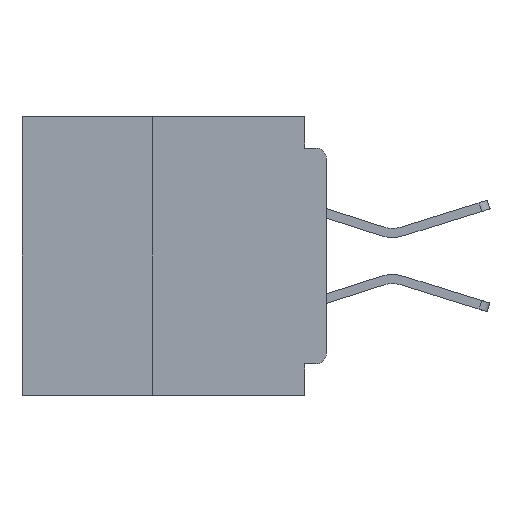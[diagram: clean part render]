
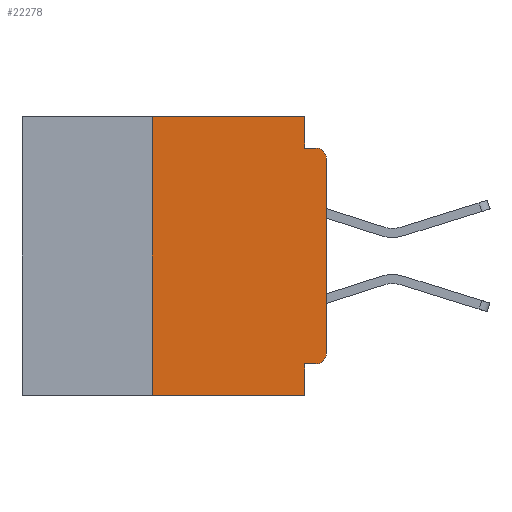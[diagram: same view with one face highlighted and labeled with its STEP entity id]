
A CAD part, left-side view. The second image highlights one B-rep face of the part: STEP entity #22278.
In plain terms, the highlighted planar face has unit normal (-1, 0, 0).
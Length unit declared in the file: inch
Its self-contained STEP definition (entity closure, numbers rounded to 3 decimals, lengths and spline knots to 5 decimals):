
#838 = DIRECTION ( 'NONE',  ( 0., 0., -1. ) ) ;
#1264 = DIRECTION ( 'NONE',  ( -1., 0., 0. ) ) ;
#1279 = VECTOR ( 'NONE', #4984, 39.37008 ) ;
#2149 = VERTEX_POINT ( 'NONE', #19976 ) ;
#2242 = AXIS2_PLACEMENT_3D ( 'NONE', #22116, #1264, #25553 ) ;
#2378 = ORIENTED_EDGE ( 'NONE', *, *, #42520, .T. ) ;
#2770 = VECTOR ( 'NONE', #7471, 39.37008 ) ;
#3563 = CARTESIAN_POINT ( 'NONE',  ( 0., 0., -0.34 ) ) ;
#3921 = CARTESIAN_POINT ( 'NONE',  ( 0., 0., -0.355 ) ) ;
#4330 = ORIENTED_EDGE ( 'NONE', *, *, #10132, .F. ) ;
#4984 = DIRECTION ( 'NONE',  ( 0., -1., 0. ) ) ;
#5129 = DIRECTION ( 'NONE',  ( 1., 0., 0. ) ) ;
#6681 = DIRECTION ( 'NONE',  ( 0., 0., -1. ) ) ;
#6884 = LINE ( 'NONE', #18357, #33269 ) ;
#7471 = DIRECTION ( 'NONE',  ( 0., 1., 0. ) ) ;
#7652 = DIRECTION ( 'NONE',  ( -1., 0., 0. ) ) ;
#9373 = CARTESIAN_POINT ( 'NONE',  ( 0., 0.437, 0. ) ) ;
#9387 = CARTESIAN_POINT ( 'NONE',  ( 0., 0.015, -0.045 ) ) ;
#9843 = ORIENTED_EDGE ( 'NONE', *, *, #18366, .F. ) ;
#10132 = EDGE_CURVE ( 'NONE', #31865, #11910, #21342, .T. ) ;
#10549 = LINE ( 'NONE', #25743, #36832 ) ;
#10996 = EDGE_CURVE ( 'NONE', #33162, #15261, #13133, .T. ) ;
#11572 = LINE ( 'NONE', #27353, #28836 ) ;
#11817 = CARTESIAN_POINT ( 'NONE',  ( 0., 0.437, -0.4 ) ) ;
#11910 = VERTEX_POINT ( 'NONE', #9387 ) ;
#11951 = DIRECTION ( 'NONE',  ( 0., -1., 0. ) ) ;
#12025 = VERTEX_POINT ( 'NONE', #23714 ) ;
#12152 = VECTOR ( 'NONE', #11951, 39.37008 ) ;
#12758 = CARTESIAN_POINT ( 'NONE',  ( 0., 0., 0. ) ) ;
#13133 = LINE ( 'NONE', #3921, #2770 ) ;
#15261 = VERTEX_POINT ( 'NONE', #28541 ) ;
#15314 = ORIENTED_EDGE ( 'NONE', *, *, #25732, .T. ) ;
#15579 = VECTOR ( 'NONE', #16210, 39.37008 ) ;
#15682 = ORIENTED_EDGE ( 'NONE', *, *, #27610, .F. ) ;
#16181 = EDGE_CURVE ( 'NONE', #16954, #34588, #42872, .T. ) ;
#16210 = DIRECTION ( 'NONE',  ( 0., 0., 1. ) ) ;
#16509 = AXIS2_PLACEMENT_3D ( 'NONE', #28320, #7652, #31721 ) ;
#16954 = VERTEX_POINT ( 'NONE', #3563 ) ;
#17645 = ORIENTED_EDGE ( 'NONE', *, *, #38196, .F. ) ;
#18357 = CARTESIAN_POINT ( 'NONE',  ( 0., 0.031, 0. ) ) ;
#18366 = EDGE_CURVE ( 'NONE', #2149, #34542, #10549, .T. ) ;
#18877 = CARTESIAN_POINT ( 'NONE',  ( 0., 0.437, 0. ) ) ;
#19976 = CARTESIAN_POINT ( 'NONE',  ( 0., 0.25, -0.4 ) ) ;
#20251 = CARTESIAN_POINT ( 'NONE',  ( 0., 0.015, -0.355 ) ) ;
#21342 = LINE ( 'NONE', #42631, #12152 ) ;
#22116 = CARTESIAN_POINT ( 'NONE',  ( 0., 0.015, -0.34 ) ) ;
#22278 = ADVANCED_FACE ( 'NONE', ( #40964 ), #22399, .F. ) ;
#22399 = PLANE ( 'NONE',  #28294 ) ;
#23239 = CARTESIAN_POINT ( 'NONE',  ( 0., 0.25, 0. ) ) ;
#23714 = CARTESIAN_POINT ( 'NONE',  ( 0., 0.031, 0. ) ) ;
#25370 = CIRCLE ( 'NONE', #2242, 0.015 ) ;
#25553 = DIRECTION ( 'NONE',  ( 0., 0., -1. ) ) ;
#25732 = EDGE_CURVE ( 'NONE', #34588, #11910, #39568, .T. ) ;
#25743 = CARTESIAN_POINT ( 'NONE',  ( 0., 0.25, -0.4 ) ) ;
#27353 = CARTESIAN_POINT ( 'NONE',  ( 0., 0.031, -0.4 ) ) ;
#27610 = EDGE_CURVE ( 'NONE', #12025, #31865, #6884, .T. ) ;
#28008 = VECTOR ( 'NONE', #33406, 39.37008 ) ;
#28294 = AXIS2_PLACEMENT_3D ( 'NONE', #18877, #5129, #29285 ) ;
#28320 = CARTESIAN_POINT ( 'NONE',  ( 0., 0.015, -0.06 ) ) ;
#28541 = CARTESIAN_POINT ( 'NONE',  ( 0., 0.031, -0.355 ) ) ;
#28836 = VECTOR ( 'NONE', #6681, 39.37008 ) ;
#29285 = DIRECTION ( 'NONE',  ( 0., 0., -1. ) ) ;
#29994 = LINE ( 'NONE', #11817, #1279 ) ;
#30107 = CARTESIAN_POINT ( 'NONE',  ( 0., 0.031, -0.045 ) ) ;
#31554 = CARTESIAN_POINT ( 'NONE',  ( 0., 0.031, -0.4 ) ) ;
#31721 = DIRECTION ( 'NONE',  ( 0., 0., -1. ) ) ;
#31865 = VERTEX_POINT ( 'NONE', #30107 ) ;
#32017 = ORIENTED_EDGE ( 'NONE', *, *, #35300, .F. ) ;
#33162 = VERTEX_POINT ( 'NONE', #20251 ) ;
#33269 = VECTOR ( 'NONE', #838, 39.37008 ) ;
#33406 = DIRECTION ( 'NONE',  ( 0., -1., 0. ) ) ;
#34542 = VERTEX_POINT ( 'NONE', #23239 ) ;
#34588 = VERTEX_POINT ( 'NONE', #40754 ) ;
#35300 = EDGE_CURVE ( 'NONE', #15261, #39075, #11572, .T. ) ;
#36827 = ORIENTED_EDGE ( 'NONE', *, *, #16181, .T. ) ;
#36832 = VECTOR ( 'NONE', #42811, 39.37008 ) ;
#37032 = LINE ( 'NONE', #9373, #28008 ) ;
#38045 = ORIENTED_EDGE ( 'NONE', *, *, #44359, .T. ) ;
#38196 = EDGE_CURVE ( 'NONE', #34542, #12025, #37032, .T. ) ;
#39075 = VERTEX_POINT ( 'NONE', #31554 ) ;
#39140 = EDGE_LOOP ( 'NONE', ( #36827, #15314, #4330, #15682, #17645, #9843, #38045, #32017, #42740, #2378 ) ) ;
#39568 = CIRCLE ( 'NONE', #16509, 0.015 ) ;
#40754 = CARTESIAN_POINT ( 'NONE',  ( 0., 0., -0.06 ) ) ;
#40964 = FACE_OUTER_BOUND ( 'NONE', #39140, .T. ) ;
#42520 = EDGE_CURVE ( 'NONE', #33162, #16954, #25370, .T. ) ;
#42631 = CARTESIAN_POINT ( 'NONE',  ( 0., 0., -0.045 ) ) ;
#42740 = ORIENTED_EDGE ( 'NONE', *, *, #10996, .F. ) ;
#42811 = DIRECTION ( 'NONE',  ( 0., 0., 1. ) ) ;
#42872 = LINE ( 'NONE', #12758, #15579 ) ;
#44359 = EDGE_CURVE ( 'NONE', #2149, #39075, #29994, .T. ) ;
